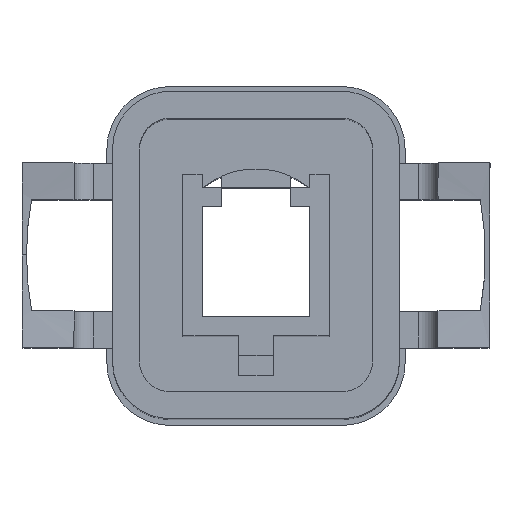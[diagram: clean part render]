
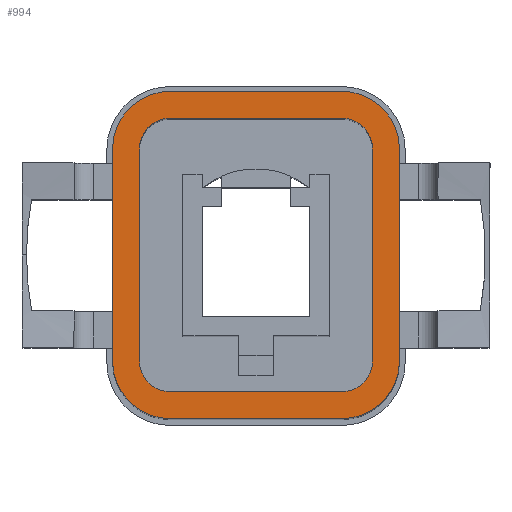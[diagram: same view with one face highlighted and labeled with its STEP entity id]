
A CAD part, top view. The second image highlights one B-rep face of the part: STEP entity #994.
In plain terms, the highlighted planar face has unit normal (0, 0, 1).
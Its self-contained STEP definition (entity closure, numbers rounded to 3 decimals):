
#46 = CARTESIAN_POINT ( 'NONE',  ( 5.95, -1.5, 0. ) ) ;
#48 = ORIENTED_EDGE ( 'NONE', *, *, #1710, .F. ) ;
#75 = AXIS2_PLACEMENT_3D ( 'NONE', #446, #2199, #2499 ) ;
#99 = DIRECTION ( 'NONE',  ( 0., -1., 0. ) ) ;
#157 = LINE ( 'NONE', #3625, #2969 ) ;
#200 = CARTESIAN_POINT ( 'NONE',  ( 5.95, -7.8, 0. ) ) ;
#208 = EDGE_LOOP ( 'NONE', ( #3387, #2132, #2775, #2891, #884, #3511, #2580, #48 ) ) ;
#269 = VERTEX_POINT ( 'NONE', #699 ) ;
#324 = LINE ( 'NONE', #2327, #1252 ) ;
#334 = CARTESIAN_POINT ( 'NONE',  ( 6.75, -1.5, 0. ) ) ;
#339 = VERTEX_POINT ( 'NONE', #3315 ) ;
#351 = DIRECTION ( 'NONE',  ( -1., 0., 0. ) ) ;
#380 = CIRCLE ( 'NONE', #1347, 0.8 ) ;
#404 = DIRECTION ( 'NONE',  ( 0., 0., 1. ) ) ;
#408 = EDGE_CURVE ( 'NONE', #269, #1132, #1955, .T. ) ;
#412 = VERTEX_POINT ( 'NONE', #3445 ) ;
#415 = CARTESIAN_POINT ( 'NONE',  ( 1.5, -8.5, 0. ) ) ;
#446 = CARTESIAN_POINT ( 'NONE',  ( 5.95, -1.5, 0. ) ) ;
#447 = LINE ( 'NONE', #1104, #2294 ) ;
#474 = CIRCLE ( 'NONE', #1625, 1.5 ) ;
#566 = ORIENTED_EDGE ( 'NONE', *, *, #1386, .T. ) ;
#583 = VERTEX_POINT ( 'NONE', #2319 ) ;
#587 = CARTESIAN_POINT ( 'NONE',  ( 5.95, -7., 0. ) ) ;
#622 = AXIS2_PLACEMENT_3D ( 'NONE', #1633, #3052, #798 ) ;
#699 = CARTESIAN_POINT ( 'NONE',  ( 1.5, -7.8, 0. ) ) ;
#710 = DIRECTION ( 'NONE',  ( 0., 0., 1. ) ) ;
#798 = DIRECTION ( 'NONE',  ( 0., -1., 0. ) ) ;
#867 = CIRCLE ( 'NONE', #1348, 1.5 ) ;
#877 = ORIENTED_EDGE ( 'NONE', *, *, #3478, .T. ) ;
#884 = ORIENTED_EDGE ( 'NONE', *, *, #2391, .F. ) ;
#921 = CIRCLE ( 'NONE', #622, 0.8 ) ;
#945 = DIRECTION ( 'NONE',  ( -1., 0., 0. ) ) ;
#947 = AXIS2_PLACEMENT_3D ( 'NONE', #46, #1536, #3546 ) ;
#952 = DIRECTION ( 'NONE',  ( 0., 0., -1. ) ) ;
#972 = LINE ( 'NONE', #2161, #1103 ) ;
#992 = CARTESIAN_POINT ( 'NONE',  ( 5.95, 0., 0. ) ) ;
#994 = ADVANCED_FACE ( 'NONE', ( #1231, #1539 ), #1129, .F. ) ;
#1013 = DIRECTION ( 'NONE',  ( 0., 1., 0. ) ) ;
#1082 = EDGE_CURVE ( 'NONE', #1249, #1866, #1476, .T. ) ;
#1101 = VERTEX_POINT ( 'NONE', #3032 ) ;
#1103 = VECTOR ( 'NONE', #351, 1000. ) ;
#1104 = CARTESIAN_POINT ( 'NONE',  ( 6.75, -7., 0. ) ) ;
#1118 = DIRECTION ( 'NONE',  ( 0., -1., 0. ) ) ;
#1125 = CARTESIAN_POINT ( 'NONE',  ( 1.5, -8.5, 0. ) ) ;
#1129 = PLANE ( 'NONE',  #1601 ) ;
#1132 = VERTEX_POINT ( 'NONE', #200 ) ;
#1231 = FACE_BOUND ( 'NONE', #208, .T. ) ;
#1249 = VERTEX_POINT ( 'NONE', #3419 ) ;
#1252 = VECTOR ( 'NONE', #3452, 1000. ) ;
#1263 = EDGE_CURVE ( 'NONE', #583, #1891, #474, .T. ) ;
#1278 = AXIS2_PLACEMENT_3D ( 'NONE', #587, #1741, #1118 ) ;
#1347 = AXIS2_PLACEMENT_3D ( 'NONE', #3308, #710, #3019 ) ;
#1348 = AXIS2_PLACEMENT_3D ( 'NONE', #1589, #1648, #2435 ) ;
#1361 = CARTESIAN_POINT ( 'NONE',  ( 1.5, -7.8, 0. ) ) ;
#1386 = EDGE_CURVE ( 'NONE', #1101, #1966, #324, .T. ) ;
#1390 = DIRECTION ( 'NONE',  ( 0., 1., 0. ) ) ;
#1461 = CIRCLE ( 'NONE', #1278, 0.8 ) ;
#1476 = CIRCLE ( 'NONE', #3599, 1.5 ) ;
#1480 = EDGE_CURVE ( 'NONE', #1866, #583, #2436, .T. ) ;
#1489 = EDGE_LOOP ( 'NONE', ( #2742, #3535, #1780, #566, #2982, #877, #1654, #3538 ) ) ;
#1536 = DIRECTION ( 'NONE',  ( 0., 0., 1. ) ) ;
#1539 = FACE_OUTER_BOUND ( 'NONE', #1489, .T. ) ;
#1558 = EDGE_CURVE ( 'NONE', #2155, #339, #157, .T. ) ;
#1572 = CARTESIAN_POINT ( 'NONE',  ( 0., -1.5, 0. ) ) ;
#1589 = CARTESIAN_POINT ( 'NONE',  ( 5.95, -7., 0. ) ) ;
#1601 = AXIS2_PLACEMENT_3D ( 'NONE', #2423, #952, #2138 ) ;
#1614 = CIRCLE ( 'NONE', #947, 0.8 ) ;
#1625 = AXIS2_PLACEMENT_3D ( 'NONE', #2589, #3501, #2040 ) ;
#1633 = CARTESIAN_POINT ( 'NONE',  ( 1.5, -1.5, 0. ) ) ;
#1648 = DIRECTION ( 'NONE',  ( 0., 0., 1. ) ) ;
#1654 = ORIENTED_EDGE ( 'NONE', *, *, #1082, .T. ) ;
#1710 = EDGE_CURVE ( 'NONE', #1132, #2099, #1461, .T. ) ;
#1741 = DIRECTION ( 'NONE',  ( 0., 0., 1. ) ) ;
#1780 = ORIENTED_EDGE ( 'NONE', *, *, #2541, .T. ) ;
#1866 = VERTEX_POINT ( 'NONE', #2651 ) ;
#1891 = VERTEX_POINT ( 'NONE', #415 ) ;
#1955 = LINE ( 'NONE', #1361, #2690 ) ;
#1966 = VERTEX_POINT ( 'NONE', #3332 ) ;
#2040 = DIRECTION ( 'NONE',  ( 0., 1., 0. ) ) ;
#2043 = VECTOR ( 'NONE', #99, 1000. ) ;
#2062 = VERTEX_POINT ( 'NONE', #334 ) ;
#2099 = VERTEX_POINT ( 'NONE', #2611 ) ;
#2132 = ORIENTED_EDGE ( 'NONE', *, *, #3540, .F. ) ;
#2138 = DIRECTION ( 'NONE',  ( 0., 1., 0. ) ) ;
#2155 = VERTEX_POINT ( 'NONE', #2334 ) ;
#2161 = CARTESIAN_POINT ( 'NONE',  ( 1.5, 0., 0. ) ) ;
#2199 = DIRECTION ( 'NONE',  ( 0., 0., 1. ) ) ;
#2285 = DIRECTION ( 'NONE',  ( 1., 0., 0. ) ) ;
#2294 = VECTOR ( 'NONE', #1390, 1000. ) ;
#2319 = CARTESIAN_POINT ( 'NONE',  ( 0., -7., 0. ) ) ;
#2327 = CARTESIAN_POINT ( 'NONE',  ( 7.45, -1.5, 0. ) ) ;
#2334 = CARTESIAN_POINT ( 'NONE',  ( 0.7, -1.5, 0. ) ) ;
#2391 = EDGE_CURVE ( 'NONE', #2993, #3435, #3542, .T. ) ;
#2423 = CARTESIAN_POINT ( 'NONE',  ( 1.5, -7., 0. ) ) ;
#2435 = DIRECTION ( 'NONE',  ( 0., -1., 0. ) ) ;
#2436 = LINE ( 'NONE', #1572, #2043 ) ;
#2499 = DIRECTION ( 'NONE',  ( 0., -1., 0. ) ) ;
#2530 = DIRECTION ( 'NONE',  ( 0., -1., 0. ) ) ;
#2541 = EDGE_CURVE ( 'NONE', #412, #1101, #867, .T. ) ;
#2574 = CARTESIAN_POINT ( 'NONE',  ( 5.95, -0.7, 0. ) ) ;
#2580 = ORIENTED_EDGE ( 'NONE', *, *, #2844, .F. ) ;
#2589 = CARTESIAN_POINT ( 'NONE',  ( 1.5, -7., 0. ) ) ;
#2611 = CARTESIAN_POINT ( 'NONE',  ( 6.75, -7., 0. ) ) ;
#2635 = CARTESIAN_POINT ( 'NONE',  ( 5.95, -0.7, 0. ) ) ;
#2651 = CARTESIAN_POINT ( 'NONE',  ( 0., -1.5, 0. ) ) ;
#2690 = VECTOR ( 'NONE', #2285, 1000. ) ;
#2742 = ORIENTED_EDGE ( 'NONE', *, *, #1263, .T. ) ;
#2775 = ORIENTED_EDGE ( 'NONE', *, *, #1558, .F. ) ;
#2844 = EDGE_CURVE ( 'NONE', #2099, #2062, #447, .T. ) ;
#2891 = ORIENTED_EDGE ( 'NONE', *, *, #3333, .F. ) ;
#2969 = VECTOR ( 'NONE', #2530, 1000. ) ;
#2982 = ORIENTED_EDGE ( 'NONE', *, *, #3568, .T. ) ;
#2993 = VERTEX_POINT ( 'NONE', #2574 ) ;
#3009 = EDGE_CURVE ( 'NONE', #1891, #412, #3722, .T. ) ;
#3019 = DIRECTION ( 'NONE',  ( 0., -1., 0. ) ) ;
#3032 = CARTESIAN_POINT ( 'NONE',  ( 7.45, -7., 0. ) ) ;
#3052 = DIRECTION ( 'NONE',  ( 0., 0., 1. ) ) ;
#3088 = EDGE_CURVE ( 'NONE', #2062, #2993, #1614, .T. ) ;
#3163 = CIRCLE ( 'NONE', #75, 1.5 ) ;
#3193 = DIRECTION ( 'NONE',  ( 1., 0., 0. ) ) ;
#3250 = VECTOR ( 'NONE', #3193, 1000. ) ;
#3254 = CARTESIAN_POINT ( 'NONE',  ( 1.5, -0.7, 0. ) ) ;
#3308 = CARTESIAN_POINT ( 'NONE',  ( 1.5, -7., 0. ) ) ;
#3315 = CARTESIAN_POINT ( 'NONE',  ( 0.7, -7., 0. ) ) ;
#3332 = CARTESIAN_POINT ( 'NONE',  ( 7.45, -1.5, 0. ) ) ;
#3333 = EDGE_CURVE ( 'NONE', #3435, #2155, #921, .T. ) ;
#3387 = ORIENTED_EDGE ( 'NONE', *, *, #408, .F. ) ;
#3413 = VECTOR ( 'NONE', #945, 1000. ) ;
#3419 = CARTESIAN_POINT ( 'NONE',  ( 1.5, 0., 0. ) ) ;
#3435 = VERTEX_POINT ( 'NONE', #3254 ) ;
#3445 = CARTESIAN_POINT ( 'NONE',  ( 5.95, -8.5, 0. ) ) ;
#3452 = DIRECTION ( 'NONE',  ( 0., 1., 0. ) ) ;
#3478 = EDGE_CURVE ( 'NONE', #3539, #1249, #972, .T. ) ;
#3501 = DIRECTION ( 'NONE',  ( 0., 0., 1. ) ) ;
#3511 = ORIENTED_EDGE ( 'NONE', *, *, #3088, .F. ) ;
#3535 = ORIENTED_EDGE ( 'NONE', *, *, #3009, .T. ) ;
#3538 = ORIENTED_EDGE ( 'NONE', *, *, #1480, .T. ) ;
#3539 = VERTEX_POINT ( 'NONE', #992 ) ;
#3540 = EDGE_CURVE ( 'NONE', #339, #269, #380, .T. ) ;
#3542 = LINE ( 'NONE', #2635, #3413 ) ;
#3546 = DIRECTION ( 'NONE',  ( 0., -1., 0. ) ) ;
#3568 = EDGE_CURVE ( 'NONE', #1966, #3539, #3163, .T. ) ;
#3589 = CARTESIAN_POINT ( 'NONE',  ( 1.5, -1.5, 0. ) ) ;
#3599 = AXIS2_PLACEMENT_3D ( 'NONE', #3589, #404, #1013 ) ;
#3625 = CARTESIAN_POINT ( 'NONE',  ( 0.7, -1.5, 0. ) ) ;
#3722 = LINE ( 'NONE', #1125, #3250 ) ;
